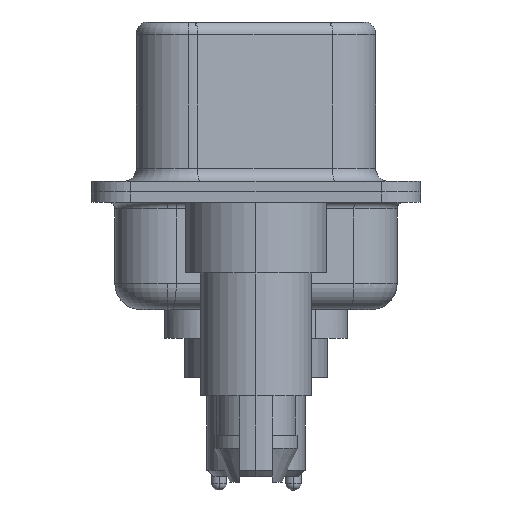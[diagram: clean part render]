
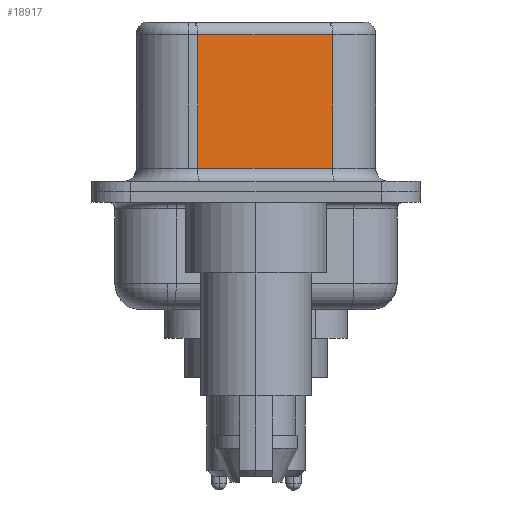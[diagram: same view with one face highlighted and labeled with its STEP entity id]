
A CAD part, left-side view. The second image highlights one B-rep face of the part: STEP entity #18917.
In plain terms, the highlighted planar face has unit normal (-0.985, -0.174, 0).
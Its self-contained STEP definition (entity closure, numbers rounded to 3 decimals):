
#17 = LINE ( 'NONE', #12082, #9964 ) ;
#510 = DIRECTION ( 'NONE',  ( -0.174, 0.985, 0. ) ) ;
#1044 = CARTESIAN_POINT ( 'NONE',  ( 4.58, -2.927, 0.9 ) ) ;
#1575 = AXIS2_PLACEMENT_3D ( 'NONE', #3225, #6957, #19951 ) ;
#3225 = CARTESIAN_POINT ( 'NONE',  ( 4.58, -2.927, 6.52 ) ) ;
#4044 = EDGE_CURVE ( 'NONE', #11174, #17474, #17, .T. ) ;
#4702 = DIRECTION ( 'NONE',  ( 0., 0., -1. ) ) ;
#4780 = VERTEX_POINT ( 'NONE', #7935 ) ;
#4853 = ORIENTED_EDGE ( 'NONE', *, *, #23267, .T. ) ;
#5017 = CARTESIAN_POINT ( 'NONE',  ( 3.67, 2.233, 6.02 ) ) ;
#5608 = ORIENTED_EDGE ( 'NONE', *, *, #11809, .F. ) ;
#6957 = DIRECTION ( 'NONE',  ( 0.985, 0.174, 0. ) ) ;
#7935 = CARTESIAN_POINT ( 'NONE',  ( 3.67, 2.233, 0.9 ) ) ;
#8302 = CARTESIAN_POINT ( 'NONE',  ( 3.67, 2.233, 6.52 ) ) ;
#9193 = VECTOR ( 'NONE', #17058, 1000. ) ;
#9566 = CARTESIAN_POINT ( 'NONE',  ( 4.58, -2.927, 6.52 ) ) ;
#9964 = VECTOR ( 'NONE', #510, 1000. ) ;
#10734 = ORIENTED_EDGE ( 'NONE', *, *, #4044, .T. ) ;
#11005 = CARTESIAN_POINT ( 'NONE',  ( 4.58, -2.927, 6.02 ) ) ;
#11174 = VERTEX_POINT ( 'NONE', #11005 ) ;
#11809 = EDGE_CURVE ( 'NONE', #11174, #18830, #19732, .T. ) ;
#12082 = CARTESIAN_POINT ( 'NONE',  ( 4.58, -2.927, 6.02 ) ) ;
#12377 = CARTESIAN_POINT ( 'NONE',  ( 4.58, -2.927, 0.9 ) ) ;
#12448 = PLANE ( 'NONE',  #1575 ) ;
#13012 = LINE ( 'NONE', #8302, #22416 ) ;
#13200 = EDGE_CURVE ( 'NONE', #4780, #18830, #19361, .T. ) ;
#13771 = VECTOR ( 'NONE', #21814, 1000. ) ;
#17058 = DIRECTION ( 'NONE',  ( 0., 0., -1. ) ) ;
#17474 = VERTEX_POINT ( 'NONE', #5017 ) ;
#18830 = VERTEX_POINT ( 'NONE', #1044 ) ;
#18917 = ADVANCED_FACE ( 'NONE', ( #20511 ), #12448, .F. ) ;
#19361 = LINE ( 'NONE', #12377, #13771 ) ;
#19732 = LINE ( 'NONE', #9566, #9193 ) ;
#19951 = DIRECTION ( 'NONE',  ( -0.174, 0.985, 0. ) ) ;
#20271 = EDGE_LOOP ( 'NONE', ( #5608, #10734, #4853, #23257 ) ) ;
#20511 = FACE_OUTER_BOUND ( 'NONE', #20271, .T. ) ;
#21814 = DIRECTION ( 'NONE',  ( 0.174, -0.985, 0. ) ) ;
#22416 = VECTOR ( 'NONE', #4702, 1000. ) ;
#23257 = ORIENTED_EDGE ( 'NONE', *, *, #13200, .T. ) ;
#23267 = EDGE_CURVE ( 'NONE', #17474, #4780, #13012, .T. ) ;
